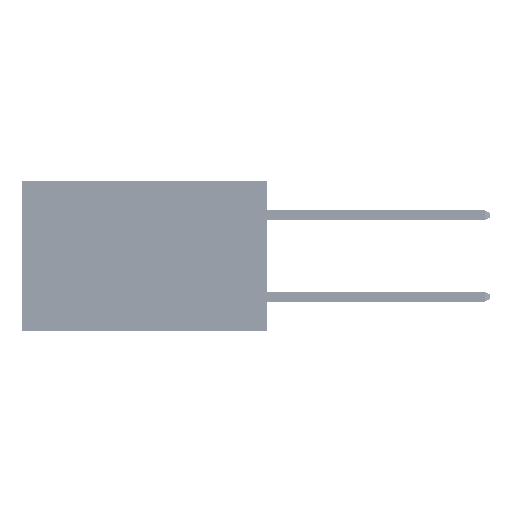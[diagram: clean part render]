
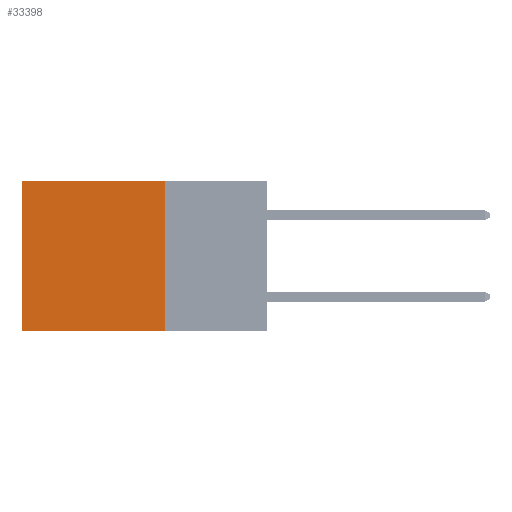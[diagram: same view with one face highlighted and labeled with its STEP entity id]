
A CAD part, left-side view. The second image highlights one B-rep face of the part: STEP entity #33398.
In plain terms, the highlighted planar face has unit normal (-1, 0, 0).
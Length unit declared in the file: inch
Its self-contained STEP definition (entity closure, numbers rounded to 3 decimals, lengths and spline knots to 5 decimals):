
#434 = ORIENTED_EDGE ( 'NONE', *, *, #24766, .F. ) ;
#3492 = DIRECTION ( 'NONE',  ( 0., 0., -1. ) ) ;
#3541 = CARTESIAN_POINT ( 'NONE',  ( 0.2875, 0.6, 0. ) ) ;
#5855 = CARTESIAN_POINT ( 'NONE',  ( 0.2875, 0.25, -0.37 ) ) ;
#6496 = DIRECTION ( 'NONE',  ( 0., 1., 0. ) ) ;
#7626 = DIRECTION ( 'NONE',  ( 0., 1., 0. ) ) ;
#9581 = CARTESIAN_POINT ( 'NONE',  ( 0.2875, 0.25, 0. ) ) ;
#10978 = CARTESIAN_POINT ( 'NONE',  ( 0.2875, 0.6, -0.37 ) ) ;
#11496 = VECTOR ( 'NONE', #7626, 39.37008 ) ;
#12180 = EDGE_CURVE ( 'NONE', #28395, #27383, #19105, .T. ) ;
#13113 = FACE_OUTER_BOUND ( 'NONE', #16132, .T. ) ;
#13783 = PLANE ( 'NONE',  #39505 ) ;
#14129 = CARTESIAN_POINT ( 'NONE',  ( 0.2875, 0.25, 0. ) ) ;
#15544 = CARTESIAN_POINT ( 'NONE',  ( 0.2875, 0.25, -0.37 ) ) ;
#16132 = EDGE_LOOP ( 'NONE', ( #16533, #42466, #434, #41049 ) ) ;
#16533 = ORIENTED_EDGE ( 'NONE', *, *, #23883, .T. ) ;
#19105 = LINE ( 'NONE', #9581, #45020 ) ;
#23883 = EDGE_CURVE ( 'NONE', #27383, #27415, #43453, .T. ) ;
#24766 = EDGE_CURVE ( 'NONE', #28395, #28680, #28913, .T. ) ;
#27383 = VERTEX_POINT ( 'NONE', #3541 ) ;
#27415 = VERTEX_POINT ( 'NONE', #10978 ) ;
#28395 = VERTEX_POINT ( 'NONE', #35073 ) ;
#28680 = VERTEX_POINT ( 'NONE', #5855 ) ;
#28913 = LINE ( 'NONE', #44092, #36175 ) ;
#29010 = VECTOR ( 'NONE', #42394, 39.37008 ) ;
#31123 = CARTESIAN_POINT ( 'NONE',  ( 0.2875, 0.6, 0. ) ) ;
#33398 = ADVANCED_FACE ( 'NONE', ( #13113 ), #13783, .F. ) ;
#35073 = CARTESIAN_POINT ( 'NONE',  ( 0.2875, 0.25, 0. ) ) ;
#36175 = VECTOR ( 'NONE', #40396, 39.37008 ) ;
#39505 = AXIS2_PLACEMENT_3D ( 'NONE', #14129, #41060, #3492 ) ;
#40396 = DIRECTION ( 'NONE',  ( 0., 0., -1. ) ) ;
#41049 = ORIENTED_EDGE ( 'NONE', *, *, #12180, .T. ) ;
#41060 = DIRECTION ( 'NONE',  ( 1., 0., 0. ) ) ;
#42394 = DIRECTION ( 'NONE',  ( 0., 0., -1. ) ) ;
#42466 = ORIENTED_EDGE ( 'NONE', *, *, #45636, .F. ) ;
#43453 = LINE ( 'NONE', #31123, #29010 ) ;
#44092 = CARTESIAN_POINT ( 'NONE',  ( 0.2875, 0.25, 0. ) ) ;
#45020 = VECTOR ( 'NONE', #6496, 39.37008 ) ;
#45636 = EDGE_CURVE ( 'NONE', #28680, #27415, #45846, .T. ) ;
#45846 = LINE ( 'NONE', #15544, #11496 ) ;
